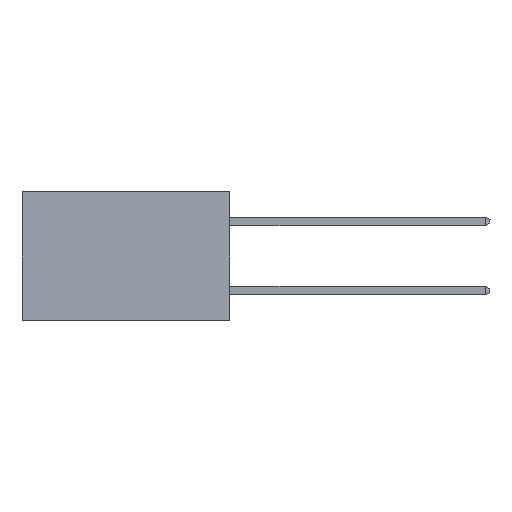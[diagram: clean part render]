
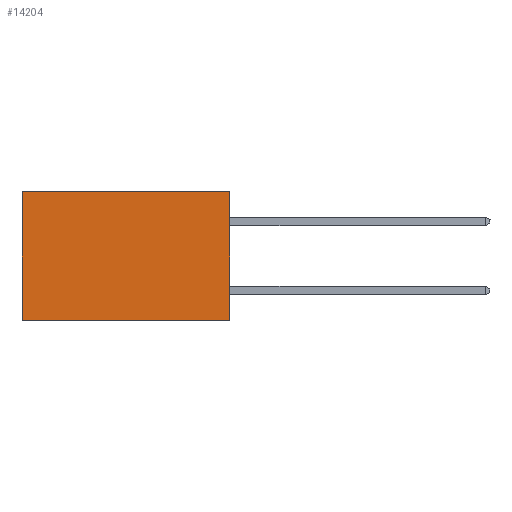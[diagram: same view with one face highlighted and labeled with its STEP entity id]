
A CAD part, left-side view. The second image highlights one B-rep face of the part: STEP entity #14204.
In plain terms, the highlighted planar face has unit normal (-1, 0, 0).
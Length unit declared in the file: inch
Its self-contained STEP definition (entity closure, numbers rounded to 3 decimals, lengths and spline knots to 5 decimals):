
#744 = ORIENTED_EDGE ( 'NONE', *, *, #11982, .T. ) ;
#1425 = VERTEX_POINT ( 'NONE', #18007 ) ;
#1479 = CARTESIAN_POINT ( 'NONE',  ( 0.2615, 0., 0. ) ) ;
#1523 = ORIENTED_EDGE ( 'NONE', *, *, #7645, .F. ) ;
#2986 = CARTESIAN_POINT ( 'NONE',  ( 0.2615, 0., -0.37 ) ) ;
#5814 = VECTOR ( 'NONE', #16003, 39.37008 ) ;
#6374 = VECTOR ( 'NONE', #16922, 39.37008 ) ;
#6735 = CARTESIAN_POINT ( 'NONE',  ( 0.2615, 0.6, 0. ) ) ;
#6894 = LINE ( 'NONE', #2986, #5814 ) ;
#7051 = CARTESIAN_POINT ( 'NONE',  ( 0.2615, 0., -0.37 ) ) ;
#7645 = EDGE_CURVE ( 'NONE', #16121, #1425, #6894, .T. ) ;
#7933 = AXIS2_PLACEMENT_3D ( 'NONE', #7051, #10436, #19552 ) ;
#9709 = LINE ( 'NONE', #11782, #22162 ) ;
#10436 = DIRECTION ( 'NONE',  ( 1., 0., 0. ) ) ;
#11782 = CARTESIAN_POINT ( 'NONE',  ( 0.2615, 0., -0.37 ) ) ;
#11982 = EDGE_CURVE ( 'NONE', #18778, #17722, #14862, .T. ) ;
#12149 = FACE_OUTER_BOUND ( 'NONE', #15313, .T. ) ;
#12349 = CARTESIAN_POINT ( 'NONE',  ( 0.2615, 0., 0. ) ) ;
#12672 = VECTOR ( 'NONE', #19881, 39.37008 ) ;
#14204 = ADVANCED_FACE ( 'NONE', ( #12149 ), #19797, .F. ) ;
#14862 = LINE ( 'NONE', #18390, #6374 ) ;
#15313 = EDGE_LOOP ( 'NONE', ( #744, #21377, #1523, #18578 ) ) ;
#16003 = DIRECTION ( 'NONE',  ( 0., 0., -1. ) ) ;
#16121 = VERTEX_POINT ( 'NONE', #1479 ) ;
#16796 = EDGE_CURVE ( 'NONE', #16121, #18778, #21595, .T. ) ;
#16922 = DIRECTION ( 'NONE',  ( 0., 0., -1. ) ) ;
#17374 = DIRECTION ( 'NONE',  ( 0., 1., 0. ) ) ;
#17722 = VERTEX_POINT ( 'NONE', #23487 ) ;
#18007 = CARTESIAN_POINT ( 'NONE',  ( 0.2615, 0., -0.37 ) ) ;
#18390 = CARTESIAN_POINT ( 'NONE',  ( 0.2615, 0.6, -0.37 ) ) ;
#18578 = ORIENTED_EDGE ( 'NONE', *, *, #16796, .T. ) ;
#18778 = VERTEX_POINT ( 'NONE', #6735 ) ;
#19552 = DIRECTION ( 'NONE',  ( 0., 0., -1. ) ) ;
#19797 = PLANE ( 'NONE',  #7933 ) ;
#19881 = DIRECTION ( 'NONE',  ( 0., 1., 0. ) ) ;
#21377 = ORIENTED_EDGE ( 'NONE', *, *, #23958, .F. ) ;
#21595 = LINE ( 'NONE', #12349, #12672 ) ;
#22162 = VECTOR ( 'NONE', #17374, 39.37008 ) ;
#23487 = CARTESIAN_POINT ( 'NONE',  ( 0.2615, 0.6, -0.37 ) ) ;
#23958 = EDGE_CURVE ( 'NONE', #1425, #17722, #9709, .T. ) ;
